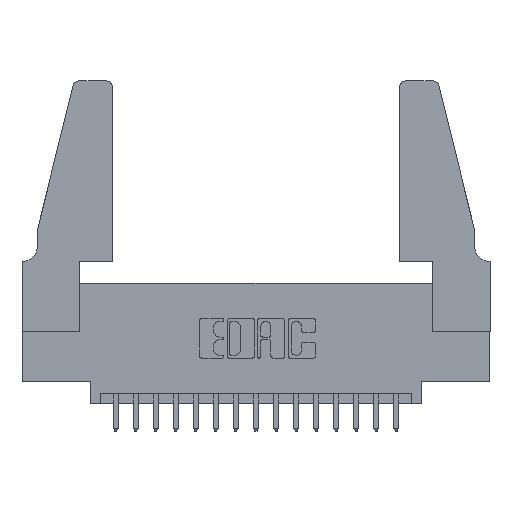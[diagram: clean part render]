
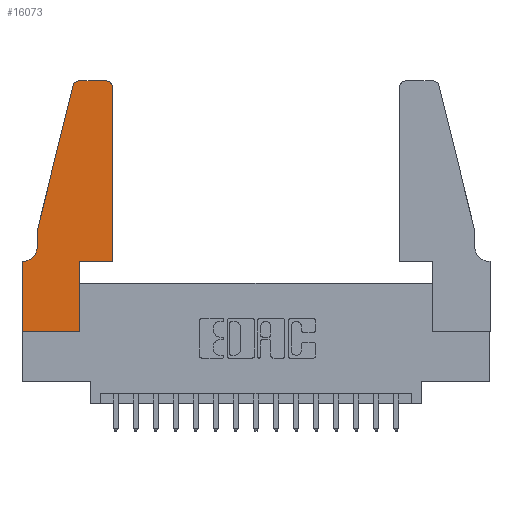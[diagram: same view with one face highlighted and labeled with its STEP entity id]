
A CAD part, top view. The second image highlights one B-rep face of the part: STEP entity #16073.
In plain terms, the highlighted planar face has unit normal (0, 0, 1).
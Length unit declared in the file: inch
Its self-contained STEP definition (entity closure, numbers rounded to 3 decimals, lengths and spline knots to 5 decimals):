
#66 = CARTESIAN_POINT ( 'NONE',  ( 0.0755, 0.35, 0.37 ) ) ;
#120 = CARTESIAN_POINT ( 'NONE',  ( 0.0755, 0.5, 0.37 ) ) ;
#323 = ORIENTED_EDGE ( 'NONE', *, *, #7630, .T. ) ;
#476 = DIRECTION ( 'NONE',  ( 1., 0., 0. ) ) ;
#704 = VERTEX_POINT ( 'NONE', #4880 ) ;
#732 = CARTESIAN_POINT ( 'NONE',  ( 0.4505, 0.35, 0.37 ) ) ;
#964 = DIRECTION ( 'NONE',  ( 1., 0., 0. ) ) ;
#1235 = ORIENTED_EDGE ( 'NONE', *, *, #7010, .T. ) ;
#1550 = LINE ( 'NONE', #4732, #11435 ) ;
#1879 = VERTEX_POINT ( 'NONE', #13971 ) ;
#1896 = EDGE_CURVE ( 'NONE', #10537, #4280, #16536, .T. ) ;
#1917 = LINE ( 'NONE', #66, #16229 ) ;
#2156 = CIRCLE ( 'NONE', #11628, 0.03 ) ;
#2202 = CARTESIAN_POINT ( 'NONE',  ( 0., 0.35, 0.37 ) ) ;
#2508 = CARTESIAN_POINT ( 'NONE',  ( 0.2605, 1.25, 0.37 ) ) ;
#2568 = CARTESIAN_POINT ( 'NONE',  ( 0.284, 1.22, 0.37 ) ) ;
#2784 = LINE ( 'NONE', #17300, #6673 ) ;
#3305 = CARTESIAN_POINT ( 'NONE',  ( 0.4505, 0.35, 0.37 ) ) ;
#3640 = CARTESIAN_POINT ( 'NONE',  ( 0.0055, 0.42, 0.37 ) ) ;
#3851 = VERTEX_POINT ( 'NONE', #7467 ) ;
#3894 = CARTESIAN_POINT ( 'NONE',  ( 0.4205, 1.25, 0.37 ) ) ;
#4280 = VERTEX_POINT ( 'NONE', #10089 ) ;
#4451 = ORIENTED_EDGE ( 'NONE', *, *, #6455, .T. ) ;
#4732 = CARTESIAN_POINT ( 'NONE',  ( 0.0755, 0.5, 0.37 ) ) ;
#4868 = LINE ( 'NONE', #15743, #17682 ) ;
#4880 = CARTESIAN_POINT ( 'NONE',  ( 0.2865, 0.35, 0.37 ) ) ;
#5437 = CARTESIAN_POINT ( 'NONE',  ( 0.2865, 0.35, 0.37 ) ) ;
#5828 = AXIS2_PLACEMENT_3D ( 'NONE', #3640, #6513, #15915 ) ;
#5910 = DIRECTION ( 'NONE',  ( 0., -1., 0. ) ) ;
#6091 = EDGE_CURVE ( 'NONE', #9988, #10537, #12191, .T. ) ;
#6455 = EDGE_CURVE ( 'NONE', #704, #11748, #13270, .T. ) ;
#6482 = PLANE ( 'NONE',  #16567 ) ;
#6513 = DIRECTION ( 'NONE',  ( 0., 0., -1. ) ) ;
#6657 = LINE ( 'NONE', #7221, #14307 ) ;
#6664 = AXIS2_PLACEMENT_3D ( 'NONE', #11386, #8645, #7392 ) ;
#6673 = VECTOR ( 'NONE', #11751, 39.37008 ) ;
#6685 = DIRECTION ( 'NONE',  ( 1., 0., 0. ) ) ;
#7010 = EDGE_CURVE ( 'NONE', #1879, #3851, #1917, .T. ) ;
#7138 = EDGE_LOOP ( 'NONE', ( #17715, #11036, #14489, #323, #14293, #1235, #9527, #7454, #10664, #4451, #16786, #16343 ) ) ;
#7221 = CARTESIAN_POINT ( 'NONE',  ( 0.0755, 0.5, 0.37 ) ) ;
#7245 = EDGE_CURVE ( 'NONE', #3851, #17052, #2784, .T. ) ;
#7380 = CARTESIAN_POINT ( 'NONE',  ( 0.4505, 1.22, 0.37 ) ) ;
#7392 = DIRECTION ( 'NONE',  ( 1., 0., 0. ) ) ;
#7454 = ORIENTED_EDGE ( 'NONE', *, *, #8893, .T. ) ;
#7467 = CARTESIAN_POINT ( 'NONE',  ( 0., 0.35, 0.37 ) ) ;
#7630 = EDGE_CURVE ( 'NONE', #8556, #11047, #6657, .T. ) ;
#7871 = DIRECTION ( 'NONE',  ( 1., 0., 0. ) ) ;
#8556 = VERTEX_POINT ( 'NONE', #120 ) ;
#8631 = VECTOR ( 'NONE', #14786, 39.37008 ) ;
#8645 = DIRECTION ( 'NONE',  ( 0., 0., 1. ) ) ;
#8893 = EDGE_CURVE ( 'NONE', #17052, #15240, #4868, .T. ) ;
#9204 = DIRECTION ( 'NONE',  ( 0., 0., 1. ) ) ;
#9395 = EDGE_CURVE ( 'NONE', #10026, #8556, #1550, .T. ) ;
#9527 = ORIENTED_EDGE ( 'NONE', *, *, #7245, .T. ) ;
#9664 = DIRECTION ( 'NONE',  ( -1., 0., 0. ) ) ;
#9988 = VERTEX_POINT ( 'NONE', #7380 ) ;
#10026 = VERTEX_POINT ( 'NONE', #17496 ) ;
#10089 = CARTESIAN_POINT ( 'NONE',  ( 0.284, 1.25, 0.37 ) ) ;
#10455 = CIRCLE ( 'NONE', #5828, 0.07 ) ;
#10537 = VERTEX_POINT ( 'NONE', #3894 ) ;
#10664 = ORIENTED_EDGE ( 'NONE', *, *, #16111, .T. ) ;
#11000 = VECTOR ( 'NONE', #13511, 39.37008 ) ;
#11036 = ORIENTED_EDGE ( 'NONE', *, *, #11296, .T. ) ;
#11047 = VERTEX_POINT ( 'NONE', #16879 ) ;
#11296 = EDGE_CURVE ( 'NONE', #4280, #10026, #2156, .T. ) ;
#11386 = CARTESIAN_POINT ( 'NONE',  ( 0.4205, 1.22, 0.37 ) ) ;
#11435 = VECTOR ( 'NONE', #11614, 39.37008 ) ;
#11614 = DIRECTION ( 'NONE',  ( -0.239, -0.971, 0. ) ) ;
#11628 = AXIS2_PLACEMENT_3D ( 'NONE', #2568, #16022, #7871 ) ;
#11748 = VERTEX_POINT ( 'NONE', #732 ) ;
#11751 = DIRECTION ( 'NONE',  ( 0., -1., 0. ) ) ;
#12191 = CIRCLE ( 'NONE', #6664, 0.03 ) ;
#12241 = LINE ( 'NONE', #5437, #8631 ) ;
#13103 = CARTESIAN_POINT ( 'NONE',  ( 0.4505, 0.35, 0.37 ) ) ;
#13270 = LINE ( 'NONE', #13103, #16460 ) ;
#13356 = EDGE_CURVE ( 'NONE', #11047, #1879, #10455, .T. ) ;
#13511 = DIRECTION ( 'NONE',  ( -1., 0., 0. ) ) ;
#13563 = CARTESIAN_POINT ( 'NONE',  ( 0., 0., 0.37 ) ) ;
#13971 = CARTESIAN_POINT ( 'NONE',  ( 0.0055, 0.35, 0.37 ) ) ;
#14293 = ORIENTED_EDGE ( 'NONE', *, *, #13356, .T. ) ;
#14307 = VECTOR ( 'NONE', #5910, 39.37008 ) ;
#14489 = ORIENTED_EDGE ( 'NONE', *, *, #9395, .T. ) ;
#14786 = DIRECTION ( 'NONE',  ( 0., 1., 0. ) ) ;
#15145 = CARTESIAN_POINT ( 'NONE',  ( 0.2865, 0., 0.37 ) ) ;
#15240 = VERTEX_POINT ( 'NONE', #15145 ) ;
#15425 = VECTOR ( 'NONE', #16986, 39.37008 ) ;
#15656 = LINE ( 'NONE', #3305, #15425 ) ;
#15743 = CARTESIAN_POINT ( 'NONE',  ( 0., 0., 0.37 ) ) ;
#15915 = DIRECTION ( 'NONE',  ( -1., 0., 0. ) ) ;
#16022 = DIRECTION ( 'NONE',  ( 0., 0., 1. ) ) ;
#16073 = ADVANCED_FACE ( 'NONE', ( #17603 ), #6482, .T. ) ;
#16111 = EDGE_CURVE ( 'NONE', #15240, #704, #12241, .T. ) ;
#16182 = EDGE_CURVE ( 'NONE', #11748, #9988, #15656, .T. ) ;
#16229 = VECTOR ( 'NONE', #9664, 39.37008 ) ;
#16343 = ORIENTED_EDGE ( 'NONE', *, *, #6091, .T. ) ;
#16460 = VECTOR ( 'NONE', #6685, 39.37008 ) ;
#16536 = LINE ( 'NONE', #2508, #11000 ) ;
#16567 = AXIS2_PLACEMENT_3D ( 'NONE', #2202, #9204, #964 ) ;
#16786 = ORIENTED_EDGE ( 'NONE', *, *, #16182, .T. ) ;
#16879 = CARTESIAN_POINT ( 'NONE',  ( 0.0755, 0.42, 0.37 ) ) ;
#16986 = DIRECTION ( 'NONE',  ( 0., 1., 0. ) ) ;
#17052 = VERTEX_POINT ( 'NONE', #13563 ) ;
#17300 = CARTESIAN_POINT ( 'NONE',  ( 0., 0., 0.37 ) ) ;
#17496 = CARTESIAN_POINT ( 'NONE',  ( 0.25487, 1.22718, 0.37 ) ) ;
#17603 = FACE_OUTER_BOUND ( 'NONE', #7138, .T. ) ;
#17682 = VECTOR ( 'NONE', #476, 39.37008 ) ;
#17715 = ORIENTED_EDGE ( 'NONE', *, *, #1896, .T. ) ;
